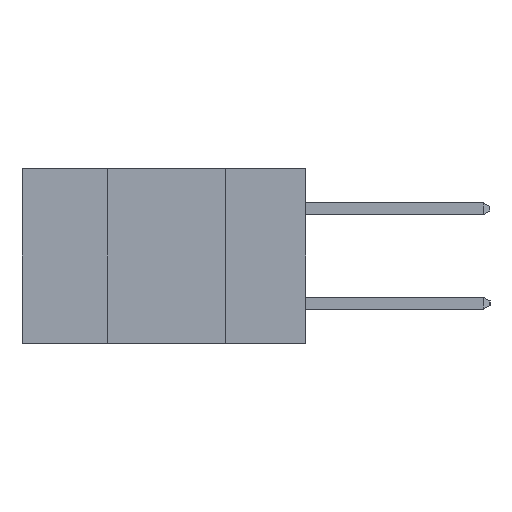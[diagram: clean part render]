
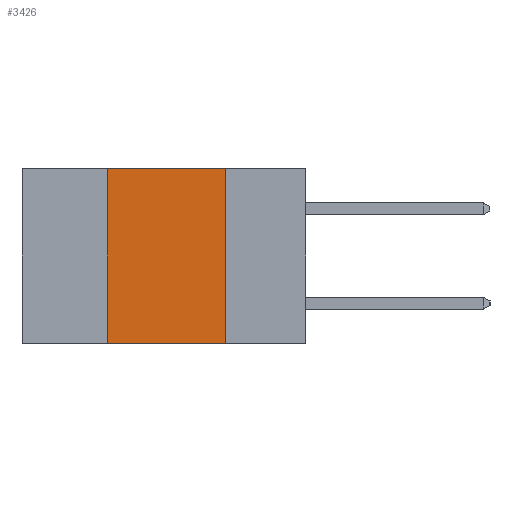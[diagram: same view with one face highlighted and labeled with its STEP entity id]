
A CAD part, left-side view. The second image highlights one B-rep face of the part: STEP entity #3426.
In plain terms, the highlighted planar face has unit normal (-1, 0, 0).
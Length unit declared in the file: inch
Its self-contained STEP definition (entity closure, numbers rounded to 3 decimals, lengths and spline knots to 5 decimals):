
#44 = ORIENTED_EDGE ( 'NONE', *, *, #9394, .T. ) ;
#89 = AXIS2_PLACEMENT_3D ( 'NONE', #12698, #2066, #8907 ) ;
#279 = VERTEX_POINT ( 'NONE', #12293 ) ;
#865 = PLANE ( 'NONE',  #89 ) ;
#890 = VECTOR ( 'NONE', #2546, 39.37008 ) ;
#1751 = CARTESIAN_POINT ( 'NONE',  ( 0., 0.6, -0.37 ) ) ;
#2066 = DIRECTION ( 'NONE',  ( 1., 0., 0. ) ) ;
#2546 = DIRECTION ( 'NONE',  ( 0., 0., 1. ) ) ;
#2849 = VERTEX_POINT ( 'NONE', #8057 ) ;
#3026 = VERTEX_POINT ( 'NONE', #3510 ) ;
#3426 = ADVANCED_FACE ( 'NONE', ( #12586 ), #865, .F. ) ;
#3510 = CARTESIAN_POINT ( 'NONE',  ( 0., 0.42, -0.37 ) ) ;
#4090 = CARTESIAN_POINT ( 'NONE',  ( 0., 0.6, 0. ) ) ;
#5296 = VECTOR ( 'NONE', #11742, 39.37008 ) ;
#6346 = LINE ( 'NONE', #11235, #890 ) ;
#6492 = CARTESIAN_POINT ( 'NONE',  ( 0., 0.17, 0. ) ) ;
#6505 = CARTESIAN_POINT ( 'NONE',  ( 0., 0.17, -0.37 ) ) ;
#6786 = VECTOR ( 'NONE', #7669, 39.37008 ) ;
#7191 = VERTEX_POINT ( 'NONE', #6492 ) ;
#7235 = DIRECTION ( 'NONE',  ( 0., 0., -1. ) ) ;
#7524 = VECTOR ( 'NONE', #7235, 39.37008 ) ;
#7669 = DIRECTION ( 'NONE',  ( 0., -1., 0. ) ) ;
#8057 = CARTESIAN_POINT ( 'NONE',  ( 0., 0.17, -0.37 ) ) ;
#8475 = EDGE_LOOP ( 'NONE', ( #11306, #12361, #12602, #44 ) ) ;
#8907 = DIRECTION ( 'NONE',  ( 0., 0., -1. ) ) ;
#9144 = EDGE_CURVE ( 'NONE', #3026, #279, #6346, .T. ) ;
#9394 = EDGE_CURVE ( 'NONE', #3026, #2849, #11877, .T. ) ;
#10388 = LINE ( 'NONE', #6505, #7524 ) ;
#10429 = EDGE_CURVE ( 'NONE', #279, #7191, #12940, .T. ) ;
#11072 = EDGE_CURVE ( 'NONE', #7191, #2849, #10388, .T. ) ;
#11235 = CARTESIAN_POINT ( 'NONE',  ( 0., 0.42, -0.37 ) ) ;
#11306 = ORIENTED_EDGE ( 'NONE', *, *, #11072, .F. ) ;
#11742 = DIRECTION ( 'NONE',  ( 0., -1., 0. ) ) ;
#11877 = LINE ( 'NONE', #1751, #6786 ) ;
#12293 = CARTESIAN_POINT ( 'NONE',  ( 0., 0.42, 0. ) ) ;
#12361 = ORIENTED_EDGE ( 'NONE', *, *, #10429, .F. ) ;
#12586 = FACE_OUTER_BOUND ( 'NONE', #8475, .T. ) ;
#12602 = ORIENTED_EDGE ( 'NONE', *, *, #9144, .F. ) ;
#12698 = CARTESIAN_POINT ( 'NONE',  ( 0., 0.6, 0. ) ) ;
#12940 = LINE ( 'NONE', #4090, #5296 ) ;
